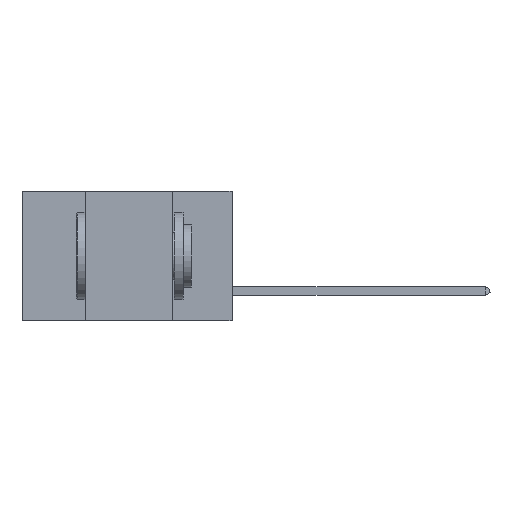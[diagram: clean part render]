
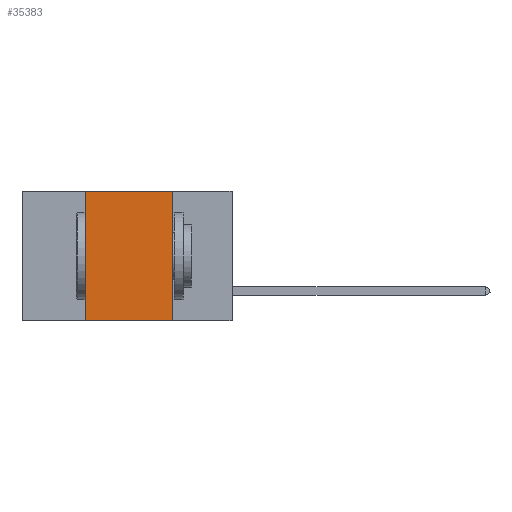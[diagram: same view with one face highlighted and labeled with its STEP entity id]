
A CAD part, left-side view. The second image highlights one B-rep face of the part: STEP entity #35383.
In plain terms, the highlighted planar face has unit normal (-1, 0, 0).
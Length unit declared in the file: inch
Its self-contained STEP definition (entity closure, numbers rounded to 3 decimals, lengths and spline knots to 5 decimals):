
#744 = VECTOR ( 'NONE', #30367, 39.37008 ) ;
#1238 = CARTESIAN_POINT ( 'NONE',  ( 0., 0.42, 0. ) ) ;
#3015 = EDGE_CURVE ( 'NONE', #9683, #6627, #20033, .T. ) ;
#3177 = EDGE_CURVE ( 'NONE', #3780, #6627, #24388, .T. ) ;
#3780 = VERTEX_POINT ( 'NONE', #7933 ) ;
#4209 = EDGE_LOOP ( 'NONE', ( #9758, #6100, #30296, #34554 ) ) ;
#5290 = CARTESIAN_POINT ( 'NONE',  ( 0., 0.17, -0.37 ) ) ;
#6100 = ORIENTED_EDGE ( 'NONE', *, *, #22847, .F. ) ;
#6627 = VERTEX_POINT ( 'NONE', #5290 ) ;
#7933 = CARTESIAN_POINT ( 'NONE',  ( 0., 0.17, 0. ) ) ;
#9683 = VERTEX_POINT ( 'NONE', #27052 ) ;
#9758 = ORIENTED_EDGE ( 'NONE', *, *, #3177, .F. ) ;
#10371 = CARTESIAN_POINT ( 'NONE',  ( 0., 0.6, 0. ) ) ;
#10624 = LINE ( 'NONE', #13504, #22591 ) ;
#11304 = PLANE ( 'NONE',  #24211 ) ;
#13504 = CARTESIAN_POINT ( 'NONE',  ( 0., 0.42, 0. ) ) ;
#17251 = FACE_OUTER_BOUND ( 'NONE', #4209, .T. ) ;
#17524 = VECTOR ( 'NONE', #35086, 39.37008 ) ;
#19247 = CARTESIAN_POINT ( 'NONE',  ( 0., 0.6, -0.37 ) ) ;
#20033 = LINE ( 'NONE', #19247, #33801 ) ;
#21672 = VERTEX_POINT ( 'NONE', #1238 ) ;
#21681 = DIRECTION ( 'NONE',  ( 0., -1., 0. ) ) ;
#22591 = VECTOR ( 'NONE', #32524, 39.37008 ) ;
#22847 = EDGE_CURVE ( 'NONE', #21672, #3780, #24868, .T. ) ;
#24211 = AXIS2_PLACEMENT_3D ( 'NONE', #24700, #32969, #33083 ) ;
#24270 = EDGE_CURVE ( 'NONE', #9683, #21672, #10624, .T. ) ;
#24388 = LINE ( 'NONE', #27380, #744 ) ;
#24700 = CARTESIAN_POINT ( 'NONE',  ( 0., 0.6, 0. ) ) ;
#24868 = LINE ( 'NONE', #10371, #17524 ) ;
#27052 = CARTESIAN_POINT ( 'NONE',  ( 0., 0.42, -0.37 ) ) ;
#27380 = CARTESIAN_POINT ( 'NONE',  ( 0., 0.17, 0. ) ) ;
#30296 = ORIENTED_EDGE ( 'NONE', *, *, #24270, .F. ) ;
#30367 = DIRECTION ( 'NONE',  ( 0., 0., -1. ) ) ;
#32524 = DIRECTION ( 'NONE',  ( 0., 0., 1. ) ) ;
#32969 = DIRECTION ( 'NONE',  ( 1., 0., 0. ) ) ;
#33083 = DIRECTION ( 'NONE',  ( 0., 0., -1. ) ) ;
#33801 = VECTOR ( 'NONE', #21681, 39.37008 ) ;
#34554 = ORIENTED_EDGE ( 'NONE', *, *, #3015, .T. ) ;
#35086 = DIRECTION ( 'NONE',  ( 0., -1., 0. ) ) ;
#35383 = ADVANCED_FACE ( 'NONE', ( #17251 ), #11304, .F. ) ;
